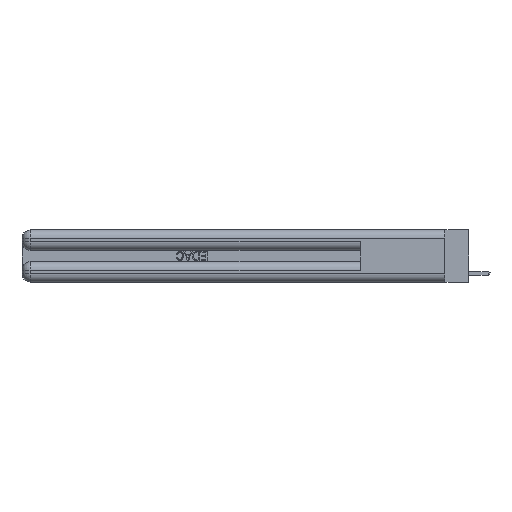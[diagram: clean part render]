
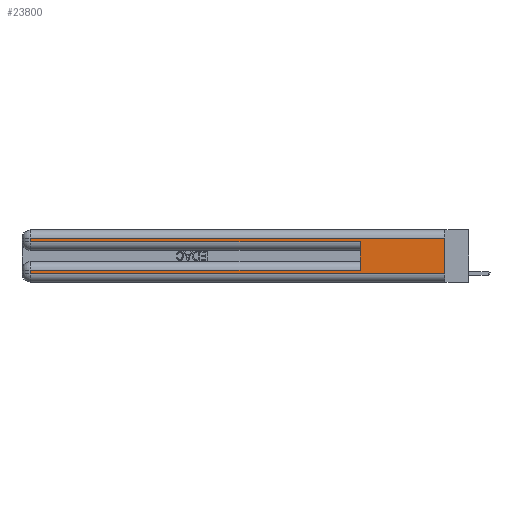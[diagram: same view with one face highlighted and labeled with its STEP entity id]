
A CAD part, left-side view. The second image highlights one B-rep face of the part: STEP entity #23800.
In plain terms, the highlighted planar face has unit normal (-1, 0, 0).
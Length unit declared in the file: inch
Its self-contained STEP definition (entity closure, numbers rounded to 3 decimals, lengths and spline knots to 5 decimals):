
#1255 = AXIS2_PLACEMENT_3D ( 'NONE', #2412, #15740, #21717 ) ;
#1427 = CARTESIAN_POINT ( 'NONE',  ( 0., 0., 0.31 ) ) ;
#1448 = VECTOR ( 'NONE', #20420, 39.37008 ) ;
#2036 = ORIENTED_EDGE ( 'NONE', *, *, #15427, .F. ) ;
#2412 = CARTESIAN_POINT ( 'NONE',  ( 0., 0., 0.37 ) ) ;
#3731 = CARTESIAN_POINT ( 'NONE',  ( 0., 2.94, 0.06 ) ) ;
#5060 = LINE ( 'NONE', #9135, #20164 ) ;
#5200 = VERTEX_POINT ( 'NONE', #3731 ) ;
#5276 = DIRECTION ( 'NONE',  ( 0., -1., 0. ) ) ;
#5546 = ORIENTED_EDGE ( 'NONE', *, *, #8429, .T. ) ;
#5706 = DIRECTION ( 'NONE',  ( 0., 0., 1. ) ) ;
#5993 = ORIENTED_EDGE ( 'NONE', *, *, #7365, .T. ) ;
#6777 = CARTESIAN_POINT ( 'NONE',  ( 0., 0.6, 0.285 ) ) ;
#6919 = CARTESIAN_POINT ( 'NONE',  ( 0., 0., 0.31 ) ) ;
#7365 = EDGE_CURVE ( 'NONE', #16364, #20007, #16615, .T. ) ;
#7534 = LINE ( 'NONE', #14104, #13930 ) ;
#7798 = VECTOR ( 'NONE', #5706, 39.37008 ) ;
#8401 = DIRECTION ( 'NONE',  ( 0., 0., -1. ) ) ;
#8429 = EDGE_CURVE ( 'NONE', #20007, #21469, #5060, .T. ) ;
#9135 = CARTESIAN_POINT ( 'NONE',  ( 0., 2.94, 0.37 ) ) ;
#9417 = CARTESIAN_POINT ( 'NONE',  ( 0., 0., 0.085 ) ) ;
#10417 = CARTESIAN_POINT ( 'NONE',  ( 0., 2.94, 0.37 ) ) ;
#10546 = LINE ( 'NONE', #11503, #7798 ) ;
#11302 = ORIENTED_EDGE ( 'NONE', *, *, #17597, .T. ) ;
#11325 = VERTEX_POINT ( 'NONE', #21558 ) ;
#11503 = CARTESIAN_POINT ( 'NONE',  ( 0., 0.6, 0.145 ) ) ;
#11838 = EDGE_LOOP ( 'NONE', ( #2036, #5993, #5546, #16041, #16634, #16600, #18097, #11302 ) ) ;
#12518 = VECTOR ( 'NONE', #17464, 39.37008 ) ;
#13142 = LINE ( 'NONE', #20829, #20960 ) ;
#13930 = VECTOR ( 'NONE', #8401, 39.37008 ) ;
#13983 = PLANE ( 'NONE',  #1255 ) ;
#14104 = CARTESIAN_POINT ( 'NONE',  ( 0., 0., 0.37 ) ) ;
#15123 = EDGE_CURVE ( 'NONE', #21469, #23953, #13142, .T. ) ;
#15386 = VECTOR ( 'NONE', #16088, 39.37008 ) ;
#15427 = EDGE_CURVE ( 'NONE', #16364, #24584, #7534, .T. ) ;
#15740 = DIRECTION ( 'NONE',  ( 1., 0., 0. ) ) ;
#16041 = ORIENTED_EDGE ( 'NONE', *, *, #15123, .T. ) ;
#16088 = DIRECTION ( 'NONE',  ( 0., 0., -1. ) ) ;
#16364 = VERTEX_POINT ( 'NONE', #1427 ) ;
#16600 = ORIENTED_EDGE ( 'NONE', *, *, #23595, .T. ) ;
#16615 = LINE ( 'NONE', #6919, #1448 ) ;
#16634 = ORIENTED_EDGE ( 'NONE', *, *, #21271, .F. ) ;
#16718 = CARTESIAN_POINT ( 'NONE',  ( 0., 2.94, 0.31 ) ) ;
#17464 = DIRECTION ( 'NONE',  ( 0., -1., 0. ) ) ;
#17597 = EDGE_CURVE ( 'NONE', #5200, #24584, #20329, .T. ) ;
#18097 = ORIENTED_EDGE ( 'NONE', *, *, #20877, .T. ) ;
#18304 = CARTESIAN_POINT ( 'NONE',  ( 0., 0., 0.06 ) ) ;
#19888 = LINE ( 'NONE', #10417, #15386 ) ;
#20007 = VERTEX_POINT ( 'NONE', #16718 ) ;
#20164 = VECTOR ( 'NONE', #24184, 39.37008 ) ;
#20329 = LINE ( 'NONE', #21240, #12518 ) ;
#20420 = DIRECTION ( 'NONE',  ( 0., 1., 0. ) ) ;
#20755 = VERTEX_POINT ( 'NONE', #25096 ) ;
#20829 = CARTESIAN_POINT ( 'NONE',  ( 0., 0., 0.285 ) ) ;
#20877 = EDGE_CURVE ( 'NONE', #11325, #5200, #19888, .T. ) ;
#20960 = VECTOR ( 'NONE', #5276, 39.37008 ) ;
#21240 = CARTESIAN_POINT ( 'NONE',  ( 0., 0., 0.06 ) ) ;
#21271 = EDGE_CURVE ( 'NONE', #20755, #23953, #10546, .T. ) ;
#21469 = VERTEX_POINT ( 'NONE', #22182 ) ;
#21558 = CARTESIAN_POINT ( 'NONE',  ( 0., 2.94, 0.085 ) ) ;
#21717 = DIRECTION ( 'NONE',  ( 0., 0., -1. ) ) ;
#22182 = CARTESIAN_POINT ( 'NONE',  ( 0., 2.94, 0.285 ) ) ;
#22783 = LINE ( 'NONE', #9417, #23401 ) ;
#23401 = VECTOR ( 'NONE', #24935, 39.37008 ) ;
#23595 = EDGE_CURVE ( 'NONE', #20755, #11325, #22783, .T. ) ;
#23800 = ADVANCED_FACE ( 'NONE', ( #24304 ), #13983, .F. ) ;
#23953 = VERTEX_POINT ( 'NONE', #6777 ) ;
#24184 = DIRECTION ( 'NONE',  ( 0., 0., -1. ) ) ;
#24304 = FACE_OUTER_BOUND ( 'NONE', #11838, .T. ) ;
#24584 = VERTEX_POINT ( 'NONE', #18304 ) ;
#24935 = DIRECTION ( 'NONE',  ( 0., 1., 0. ) ) ;
#25096 = CARTESIAN_POINT ( 'NONE',  ( 0., 0.6, 0.085 ) ) ;
